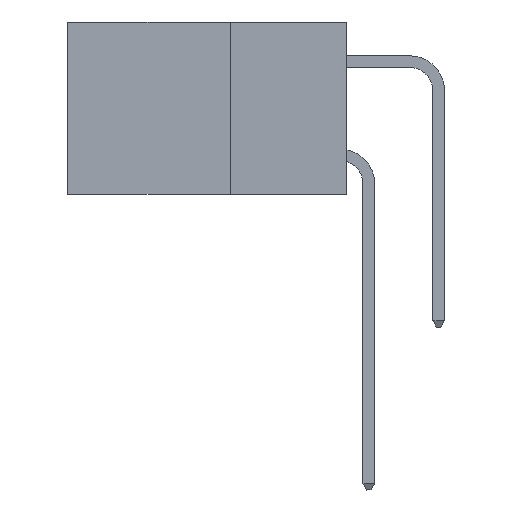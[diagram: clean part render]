
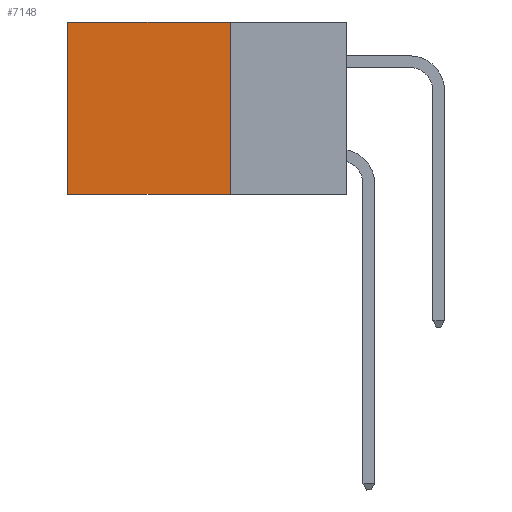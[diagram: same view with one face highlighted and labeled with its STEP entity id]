
A CAD part, left-side view. The second image highlights one B-rep face of the part: STEP entity #7148.
In plain terms, the highlighted planar face has unit normal (-1, 0, 0).
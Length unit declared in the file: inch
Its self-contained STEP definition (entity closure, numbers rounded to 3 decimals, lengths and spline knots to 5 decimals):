
#494 = DIRECTION ( 'NONE',  ( 1., 0., 0. ) ) ;
#577 = CARTESIAN_POINT ( 'NONE',  ( 0.2875, 0.25, -0.37 ) ) ;
#984 = FACE_OUTER_BOUND ( 'NONE', #22685, .T. ) ;
#1675 = DIRECTION ( 'NONE',  ( 0., 0., -1. ) ) ;
#2627 = ORIENTED_EDGE ( 'NONE', *, *, #6770, .T. ) ;
#2998 = VERTEX_POINT ( 'NONE', #18856 ) ;
#4118 = LINE ( 'NONE', #6632, #28441 ) ;
#4706 = VECTOR ( 'NONE', #16115, 39.37008 ) ;
#6153 = CARTESIAN_POINT ( 'NONE',  ( 0.2875, 0.25, -0.37 ) ) ;
#6237 = EDGE_CURVE ( 'NONE', #13363, #10190, #26160, .T. ) ;
#6632 = CARTESIAN_POINT ( 'NONE',  ( 0.2875, 0.25, 0. ) ) ;
#6770 = EDGE_CURVE ( 'NONE', #20300, #10190, #23152, .T. ) ;
#7148 = ADVANCED_FACE ( 'NONE', ( #984 ), #24024, .F. ) ;
#7162 = CARTESIAN_POINT ( 'NONE',  ( 0.2875, 0.6, -0.37 ) ) ;
#8059 = AXIS2_PLACEMENT_3D ( 'NONE', #21518, #494, #17025 ) ;
#10190 = VERTEX_POINT ( 'NONE', #7162 ) ;
#10977 = DIRECTION ( 'NONE',  ( 0., 1., 0. ) ) ;
#11938 = ORIENTED_EDGE ( 'NONE', *, *, #15794, .T. ) ;
#13363 = VERTEX_POINT ( 'NONE', #577 ) ;
#13415 = CARTESIAN_POINT ( 'NONE',  ( 0.2875, 0.6, 0. ) ) ;
#13885 = LINE ( 'NONE', #23198, #4706 ) ;
#15794 = EDGE_CURVE ( 'NONE', #2998, #20300, #13885, .T. ) ;
#16115 = DIRECTION ( 'NONE',  ( 0., 1., 0. ) ) ;
#16137 = CARTESIAN_POINT ( 'NONE',  ( 0.2875, 0.6, 0. ) ) ;
#16478 = ORIENTED_EDGE ( 'NONE', *, *, #18973, .F. ) ;
#17025 = DIRECTION ( 'NONE',  ( 0., 0., -1. ) ) ;
#18398 = VECTOR ( 'NONE', #1675, 39.37008 ) ;
#18856 = CARTESIAN_POINT ( 'NONE',  ( 0.2875, 0.25, 0. ) ) ;
#18973 = EDGE_CURVE ( 'NONE', #2998, #13363, #4118, .T. ) ;
#19158 = VECTOR ( 'NONE', #10977, 39.37008 ) ;
#20300 = VERTEX_POINT ( 'NONE', #16137 ) ;
#21518 = CARTESIAN_POINT ( 'NONE',  ( 0.2875, 0.25, 0. ) ) ;
#22685 = EDGE_LOOP ( 'NONE', ( #2627, #26819, #16478, #11938 ) ) ;
#23152 = LINE ( 'NONE', #13415, #18398 ) ;
#23198 = CARTESIAN_POINT ( 'NONE',  ( 0.2875, 0.25, 0. ) ) ;
#24024 = PLANE ( 'NONE',  #8059 ) ;
#26160 = LINE ( 'NONE', #6153, #19158 ) ;
#26819 = ORIENTED_EDGE ( 'NONE', *, *, #6237, .F. ) ;
#28441 = VECTOR ( 'NONE', #30258, 39.37008 ) ;
#30258 = DIRECTION ( 'NONE',  ( 0., 0., -1. ) ) ;
